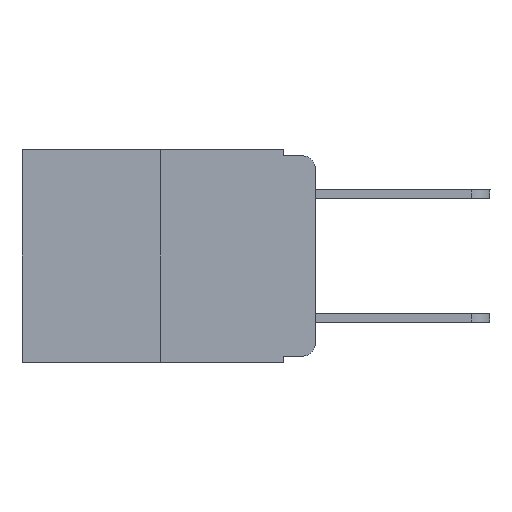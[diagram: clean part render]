
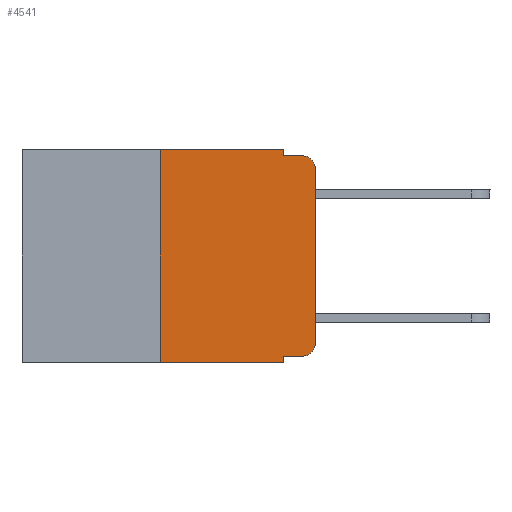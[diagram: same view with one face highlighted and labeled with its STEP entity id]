
A CAD part, left-side view. The second image highlights one B-rep face of the part: STEP entity #4541.
In plain terms, the highlighted planar face has unit normal (-1, 0, 0).
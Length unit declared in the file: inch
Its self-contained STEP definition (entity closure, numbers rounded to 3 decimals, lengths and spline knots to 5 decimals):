
#86 = CARTESIAN_POINT ( 'NONE',  ( 0., 0.051, -0.333 ) ) ;
#274 = LINE ( 'NONE', #19165, #2634 ) ;
#678 = VECTOR ( 'NONE', #6777, 39.37008 ) ;
#861 = EDGE_CURVE ( 'NONE', #16216, #6995, #9489, .T. ) ;
#1322 = LINE ( 'NONE', #7652, #19124 ) ;
#1397 = DIRECTION ( 'NONE',  ( -1., 0., 0. ) ) ;
#1444 = CARTESIAN_POINT ( 'NONE',  ( 0., 0.051, 0. ) ) ;
#1484 = EDGE_CURVE ( 'NONE', #8647, #8461, #1625, .T. ) ;
#1540 = CARTESIAN_POINT ( 'NONE',  ( 0., 0.25, 0. ) ) ;
#1625 = LINE ( 'NONE', #15353, #19283 ) ;
#2078 = EDGE_CURVE ( 'NONE', #13557, #6995, #5122, .T. ) ;
#2089 = LINE ( 'NONE', #8426, #15730 ) ;
#2259 = LINE ( 'NONE', #14916, #7209 ) ;
#2634 = VECTOR ( 'NONE', #4970, 39.37008 ) ;
#3121 = CARTESIAN_POINT ( 'NONE',  ( 0., 0.473, 0. ) ) ;
#3880 = CARTESIAN_POINT ( 'NONE',  ( 0., 0.25, -0.343 ) ) ;
#4541 = ADVANCED_FACE ( 'NONE', ( #7687 ), #9663, .F. ) ;
#4579 = ORIENTED_EDGE ( 'NONE', *, *, #20080, .T. ) ;
#4605 = CARTESIAN_POINT ( 'NONE',  ( 0., 0.25, 0. ) ) ;
#4806 = DIRECTION ( 'NONE',  ( 0., -1., 0. ) ) ;
#4874 = VECTOR ( 'NONE', #9681, 39.37008 ) ;
#4970 = DIRECTION ( 'NONE',  ( 0., 0., -1. ) ) ;
#5036 = CARTESIAN_POINT ( 'NONE',  ( 0., 0.051, -0.343 ) ) ;
#5122 = LINE ( 'NONE', #12991, #678 ) ;
#5522 = CARTESIAN_POINT ( 'NONE',  ( 0., 0.051, -0.01 ) ) ;
#5589 = VECTOR ( 'NONE', #17488, 39.37008 ) ;
#5633 = ORIENTED_EDGE ( 'NONE', *, *, #2078, .F. ) ;
#5653 = ORIENTED_EDGE ( 'NONE', *, *, #8981, .F. ) ;
#5693 = DIRECTION ( 'NONE',  ( 0., 0., 1. ) ) ;
#6307 = VERTEX_POINT ( 'NONE', #1540 ) ;
#6567 = ORIENTED_EDGE ( 'NONE', *, *, #13363, .T. ) ;
#6695 = ORIENTED_EDGE ( 'NONE', *, *, #15905, .F. ) ;
#6777 = DIRECTION ( 'NONE',  ( 0., -1., 0. ) ) ;
#6995 = VERTEX_POINT ( 'NONE', #9189 ) ;
#7085 = ORIENTED_EDGE ( 'NONE', *, *, #1484, .T. ) ;
#7209 = VECTOR ( 'NONE', #5693, 39.37008 ) ;
#7652 = CARTESIAN_POINT ( 'NONE',  ( 0., 0.051, 0. ) ) ;
#7682 = EDGE_LOOP ( 'NONE', ( #11489, #14997, #5633, #18078, #5653, #15833, #7085, #6695, #4579, #6567 ) ) ;
#7687 = FACE_OUTER_BOUND ( 'NONE', #7682, .T. ) ;
#8200 = VERTEX_POINT ( 'NONE', #18138 ) ;
#8208 = CIRCLE ( 'NONE', #20433, 0.02 ) ;
#8426 = CARTESIAN_POINT ( 'NONE',  ( 0., 0.473, 0. ) ) ;
#8461 = VERTEX_POINT ( 'NONE', #5036 ) ;
#8647 = VERTEX_POINT ( 'NONE', #3880 ) ;
#8861 = DIRECTION ( 'NONE',  ( -1., 0., 0. ) ) ;
#8981 = EDGE_CURVE ( 'NONE', #6307, #9151, #2089, .T. ) ;
#9124 = DIRECTION ( 'NONE',  ( 0., 0., -1. ) ) ;
#9151 = VERTEX_POINT ( 'NONE', #1444 ) ;
#9189 = CARTESIAN_POINT ( 'NONE',  ( 0., 0.02, -0.01 ) ) ;
#9489 = CIRCLE ( 'NONE', #16461, 0.02 ) ;
#9663 = PLANE ( 'NONE',  #13738 ) ;
#9681 = DIRECTION ( 'NONE',  ( 0., 0., 1. ) ) ;
#10663 = DIRECTION ( 'NONE',  ( 0., 0., -1. ) ) ;
#10860 = CARTESIAN_POINT ( 'NONE',  ( 0., 0., -0.03 ) ) ;
#11185 = VERTEX_POINT ( 'NONE', #86 ) ;
#11489 = ORIENTED_EDGE ( 'NONE', *, *, #17471, .T. ) ;
#12492 = CARTESIAN_POINT ( 'NONE',  ( 0., 0.051, -0.333 ) ) ;
#12756 = DIRECTION ( 'NONE',  ( 0., 0., -1. ) ) ;
#12869 = EDGE_CURVE ( 'NONE', #9151, #13557, #1322, .T. ) ;
#12991 = CARTESIAN_POINT ( 'NONE',  ( 0., 0.051, -0.01 ) ) ;
#13363 = EDGE_CURVE ( 'NONE', #18291, #8200, #8208, .T. ) ;
#13400 = CARTESIAN_POINT ( 'NONE',  ( 0., 0.02, -0.03 ) ) ;
#13557 = VERTEX_POINT ( 'NONE', #5522 ) ;
#13738 = AXIS2_PLACEMENT_3D ( 'NONE', #3121, #15782, #12756 ) ;
#14916 = CARTESIAN_POINT ( 'NONE',  ( 0., 0., 0. ) ) ;
#14997 = ORIENTED_EDGE ( 'NONE', *, *, #861, .T. ) ;
#15353 = CARTESIAN_POINT ( 'NONE',  ( 0., 0.473, -0.343 ) ) ;
#15718 = LINE ( 'NONE', #12492, #5589 ) ;
#15730 = VECTOR ( 'NONE', #4806, 39.37008 ) ;
#15782 = DIRECTION ( 'NONE',  ( 1., 0., 0. ) ) ;
#15833 = ORIENTED_EDGE ( 'NONE', *, *, #16863, .F. ) ;
#15905 = EDGE_CURVE ( 'NONE', #11185, #8461, #274, .T. ) ;
#16216 = VERTEX_POINT ( 'NONE', #10860 ) ;
#16326 = CARTESIAN_POINT ( 'NONE',  ( 0., 0.02, -0.333 ) ) ;
#16461 = AXIS2_PLACEMENT_3D ( 'NONE', #13400, #8861, #19730 ) ;
#16863 = EDGE_CURVE ( 'NONE', #8647, #6307, #19110, .T. ) ;
#17471 = EDGE_CURVE ( 'NONE', #8200, #16216, #2259, .T. ) ;
#17488 = DIRECTION ( 'NONE',  ( 0., -1., 0. ) ) ;
#18078 = ORIENTED_EDGE ( 'NONE', *, *, #12869, .F. ) ;
#18138 = CARTESIAN_POINT ( 'NONE',  ( 0., 0., -0.313 ) ) ;
#18291 = VERTEX_POINT ( 'NONE', #16326 ) ;
#18463 = DIRECTION ( 'NONE',  ( 0., -1., 0. ) ) ;
#19110 = LINE ( 'NONE', #4605, #4874 ) ;
#19124 = VECTOR ( 'NONE', #9124, 39.37008 ) ;
#19165 = CARTESIAN_POINT ( 'NONE',  ( 0., 0.051, 0. ) ) ;
#19283 = VECTOR ( 'NONE', #18463, 39.37008 ) ;
#19730 = DIRECTION ( 'NONE',  ( 0., 0., -1. ) ) ;
#20080 = EDGE_CURVE ( 'NONE', #11185, #18291, #15718, .T. ) ;
#20358 = CARTESIAN_POINT ( 'NONE',  ( 0., 0.02, -0.313 ) ) ;
#20433 = AXIS2_PLACEMENT_3D ( 'NONE', #20358, #1397, #10663 ) ;
